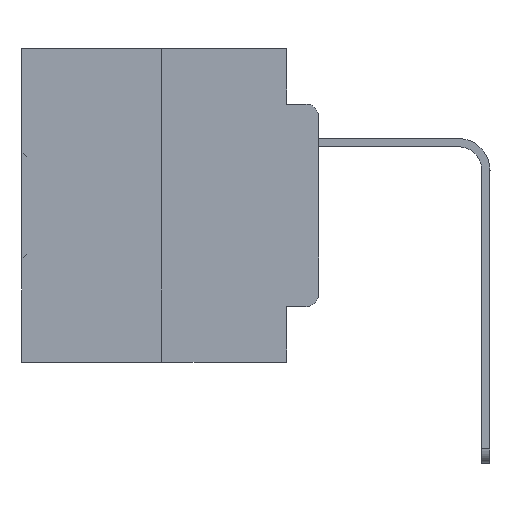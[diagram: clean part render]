
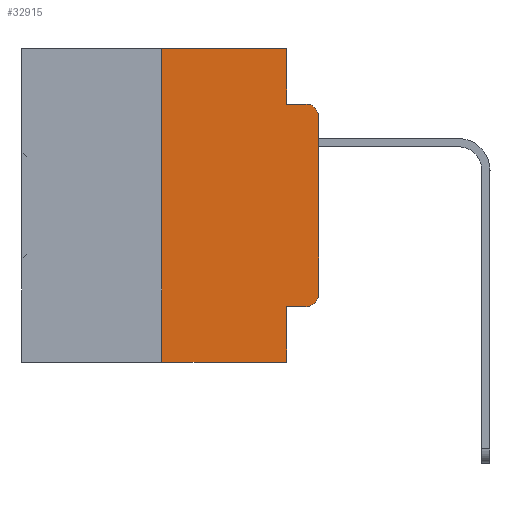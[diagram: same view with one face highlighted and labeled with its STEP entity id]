
A CAD part, left-side view. The second image highlights one B-rep face of the part: STEP entity #32915.
In plain terms, the highlighted planar face has unit normal (-1, 0, 0).
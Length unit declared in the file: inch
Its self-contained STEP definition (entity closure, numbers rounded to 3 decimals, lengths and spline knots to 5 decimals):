
#267 = ORIENTED_EDGE ( 'NONE', *, *, #28725, .T. ) ;
#789 = DIRECTION ( 'NONE',  ( 0., -1., 0. ) ) ;
#1066 = VERTEX_POINT ( 'NONE', #11009 ) ;
#1268 = DIRECTION ( 'NONE',  ( 0., 0., -1. ) ) ;
#1566 = ORIENTED_EDGE ( 'NONE', *, *, #27064, .T. ) ;
#2413 = VECTOR ( 'NONE', #28909, 39.37008 ) ;
#2446 = VERTEX_POINT ( 'NONE', #12794 ) ;
#3280 = DIRECTION ( 'NONE',  ( 0., -1., 0. ) ) ;
#3334 = EDGE_CURVE ( 'NONE', #6960, #29590, #10171, .T. ) ;
#3425 = LINE ( 'NONE', #6227, #23033 ) ;
#3730 = VERTEX_POINT ( 'NONE', #28210 ) ;
#4983 = CARTESIAN_POINT ( 'NONE',  ( 0., 0.051, -0.0885 ) ) ;
#5594 = DIRECTION ( 'NONE',  ( -1., 0., 0. ) ) ;
#6095 = VECTOR ( 'NONE', #789, 39.37008 ) ;
#6227 = CARTESIAN_POINT ( 'NONE',  ( 0., 0.25, 0. ) ) ;
#6423 = CARTESIAN_POINT ( 'NONE',  ( 0., 0.25, -0.5 ) ) ;
#6680 = EDGE_CURVE ( 'NONE', #7247, #27175, #31566, .T. ) ;
#6946 = LINE ( 'NONE', #31695, #29760 ) ;
#6960 = VERTEX_POINT ( 'NONE', #4983 ) ;
#7247 = VERTEX_POINT ( 'NONE', #22004 ) ;
#7676 = LINE ( 'NONE', #13460, #6095 ) ;
#8453 = LINE ( 'NONE', #22646, #29699 ) ;
#8534 = VERTEX_POINT ( 'NONE', #17595 ) ;
#8689 = DIRECTION ( 'NONE',  ( 0., 0., -1. ) ) ;
#10094 = CIRCLE ( 'NONE', #12698, 0.02 ) ;
#10171 = LINE ( 'NONE', #13108, #21437 ) ;
#10697 = DIRECTION ( 'NONE',  ( 0., 0., -1. ) ) ;
#11009 = CARTESIAN_POINT ( 'NONE',  ( 0., 0.25, 0. ) ) ;
#11149 = EDGE_CURVE ( 'NONE', #11886, #27175, #7676, .T. ) ;
#11175 = PLANE ( 'NONE',  #14193 ) ;
#11387 = DIRECTION ( 'NONE',  ( 1., 0., 0. ) ) ;
#11828 = DIRECTION ( 'NONE',  ( -1., 0., 0. ) ) ;
#11886 = VERTEX_POINT ( 'NONE', #6423 ) ;
#12698 = AXIS2_PLACEMENT_3D ( 'NONE', #30182, #11828, #14724 ) ;
#12794 = CARTESIAN_POINT ( 'NONE',  ( 0., 0., -0.1085 ) ) ;
#13108 = CARTESIAN_POINT ( 'NONE',  ( 0., 0.051, -0.0885 ) ) ;
#13432 = CIRCLE ( 'NONE', #22743, 0.02 ) ;
#13460 = CARTESIAN_POINT ( 'NONE',  ( 0., 0.473, -0.5 ) ) ;
#14188 = CARTESIAN_POINT ( 'NONE',  ( 0., 0.473, 0. ) ) ;
#14193 = AXIS2_PLACEMENT_3D ( 'NONE', #24070, #11387, #8689 ) ;
#14724 = DIRECTION ( 'NONE',  ( 0., 0., -1. ) ) ;
#16263 = DIRECTION ( 'NONE',  ( 0., -1., 0. ) ) ;
#17595 = CARTESIAN_POINT ( 'NONE',  ( 0., 0.051, 0. ) ) ;
#19233 = ORIENTED_EDGE ( 'NONE', *, *, #23069, .F. ) ;
#19244 = ORIENTED_EDGE ( 'NONE', *, *, #31462, .T. ) ;
#19501 = ORIENTED_EDGE ( 'NONE', *, *, #31662, .F. ) ;
#19863 = EDGE_LOOP ( 'NONE', ( #267, #21211, #26189, #19233, #28934, #19501, #30119, #24148, #1566, #19244 ) ) ;
#20278 = EDGE_CURVE ( 'NONE', #1066, #8534, #30767, .T. ) ;
#21211 = ORIENTED_EDGE ( 'NONE', *, *, #22348, .T. ) ;
#21437 = VECTOR ( 'NONE', #3280, 39.37008 ) ;
#21719 = VERTEX_POINT ( 'NONE', #32545 ) ;
#21835 = CARTESIAN_POINT ( 'NONE',  ( 0., 0.051, -0.5 ) ) ;
#22004 = CARTESIAN_POINT ( 'NONE',  ( 0., 0.051, -0.4115 ) ) ;
#22348 = EDGE_CURVE ( 'NONE', #2446, #29590, #10094, .T. ) ;
#22646 = CARTESIAN_POINT ( 'NONE',  ( 0., 0.051, 0. ) ) ;
#22743 = AXIS2_PLACEMENT_3D ( 'NONE', #23156, #5594, #10697 ) ;
#23033 = VECTOR ( 'NONE', #31637, 39.37008 ) ;
#23069 = EDGE_CURVE ( 'NONE', #8534, #6960, #8453, .T. ) ;
#23156 = CARTESIAN_POINT ( 'NONE',  ( 0., 0.02, -0.3915 ) ) ;
#24070 = CARTESIAN_POINT ( 'NONE',  ( 0., 0.473, 0. ) ) ;
#24148 = ORIENTED_EDGE ( 'NONE', *, *, #6680, .F. ) ;
#24890 = DIRECTION ( 'NONE',  ( 0., 0., -1. ) ) ;
#26152 = FACE_OUTER_BOUND ( 'NONE', #19863, .T. ) ;
#26189 = ORIENTED_EDGE ( 'NONE', *, *, #3334, .F. ) ;
#26590 = CARTESIAN_POINT ( 'NONE',  ( 0., 0.051, 0. ) ) ;
#27064 = EDGE_CURVE ( 'NONE', #7247, #21719, #6946, .T. ) ;
#27175 = VERTEX_POINT ( 'NONE', #21835 ) ;
#27516 = DIRECTION ( 'NONE',  ( 0., -1., 0. ) ) ;
#28210 = CARTESIAN_POINT ( 'NONE',  ( 0., 0., -0.3915 ) ) ;
#28725 = EDGE_CURVE ( 'NONE', #3730, #2446, #30827, .T. ) ;
#28798 = CARTESIAN_POINT ( 'NONE',  ( 0., 0., 0. ) ) ;
#28909 = DIRECTION ( 'NONE',  ( 0., 0., 1. ) ) ;
#28934 = ORIENTED_EDGE ( 'NONE', *, *, #20278, .F. ) ;
#29590 = VERTEX_POINT ( 'NONE', #30746 ) ;
#29699 = VECTOR ( 'NONE', #24890, 39.37008 ) ;
#29760 = VECTOR ( 'NONE', #16263, 39.37008 ) ;
#30119 = ORIENTED_EDGE ( 'NONE', *, *, #11149, .T. ) ;
#30182 = CARTESIAN_POINT ( 'NONE',  ( 0., 0.02, -0.1085 ) ) ;
#30746 = CARTESIAN_POINT ( 'NONE',  ( 0., 0.02, -0.0885 ) ) ;
#30767 = LINE ( 'NONE', #14188, #31577 ) ;
#30827 = LINE ( 'NONE', #28798, #2413 ) ;
#31462 = EDGE_CURVE ( 'NONE', #21719, #3730, #13432, .T. ) ;
#31566 = LINE ( 'NONE', #26590, #32728 ) ;
#31577 = VECTOR ( 'NONE', #27516, 39.37008 ) ;
#31637 = DIRECTION ( 'NONE',  ( 0., 0., 1. ) ) ;
#31662 = EDGE_CURVE ( 'NONE', #11886, #1066, #3425, .T. ) ;
#31695 = CARTESIAN_POINT ( 'NONE',  ( 0., 0.051, -0.4115 ) ) ;
#32545 = CARTESIAN_POINT ( 'NONE',  ( 0., 0.02, -0.4115 ) ) ;
#32728 = VECTOR ( 'NONE', #1268, 39.37008 ) ;
#32915 = ADVANCED_FACE ( 'NONE', ( #26152 ), #11175, .F. ) ;
